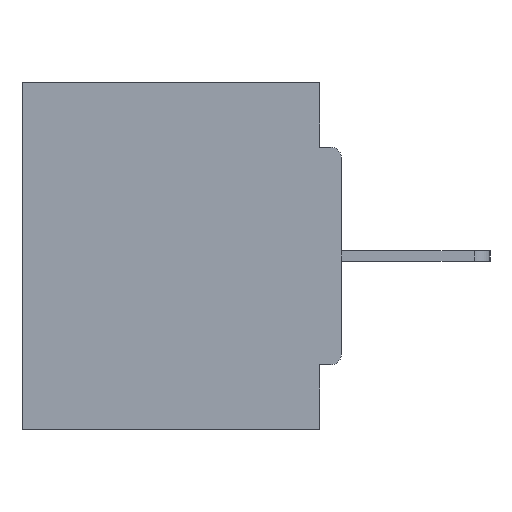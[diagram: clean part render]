
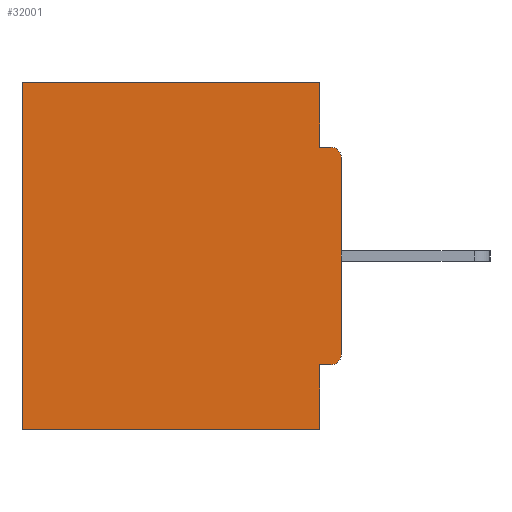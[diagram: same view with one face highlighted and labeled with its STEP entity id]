
A CAD part, left-side view. The second image highlights one B-rep face of the part: STEP entity #32001.
In plain terms, the highlighted planar face has unit normal (-1, 0, 0).
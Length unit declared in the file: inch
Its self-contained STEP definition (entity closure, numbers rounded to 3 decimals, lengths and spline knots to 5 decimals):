
#364 = DIRECTION ( 'NONE',  ( -1., 0., 0. ) ) ;
#591 = ORIENTED_EDGE ( 'NONE', *, *, #34747, .F. ) ;
#621 = ORIENTED_EDGE ( 'NONE', *, *, #23755, .F. ) ;
#860 = VERTEX_POINT ( 'NONE', #31002 ) ;
#2005 = VERTEX_POINT ( 'NONE', #24879 ) ;
#2079 = VERTEX_POINT ( 'NONE', #33691 ) ;
#2296 = VERTEX_POINT ( 'NONE', #29542 ) ;
#2443 = VECTOR ( 'NONE', #19732, 39.37008 ) ;
#3284 = ORIENTED_EDGE ( 'NONE', *, *, #6980, .F. ) ;
#3591 = CARTESIAN_POINT ( 'NONE',  ( 0.298, 0.015, -0.1085 ) ) ;
#4628 = CARTESIAN_POINT ( 'NONE',  ( 0.298, 0., -0.4065 ) ) ;
#4736 = CARTESIAN_POINT ( 'NONE',  ( 0.298, 0.015, -0.4065 ) ) ;
#5088 = EDGE_CURVE ( 'NONE', #2296, #21589, #22859, .T. ) ;
#5742 = DIRECTION ( 'NONE',  ( 0., 0., -1. ) ) ;
#5996 = CARTESIAN_POINT ( 'NONE',  ( 0.298, 0.015, -0.3915 ) ) ;
#6000 = DIRECTION ( 'NONE',  ( 1., 0., 0. ) ) ;
#6258 = EDGE_CURVE ( 'NONE', #8604, #18274, #10541, .T. ) ;
#6264 = DIRECTION ( 'NONE',  ( 0., 0., -1. ) ) ;
#6980 = EDGE_CURVE ( 'NONE', #11764, #2005, #26445, .T. ) ;
#7114 = AXIS2_PLACEMENT_3D ( 'NONE', #3591, #364, #24873 ) ;
#7462 = ORIENTED_EDGE ( 'NONE', *, *, #21615, .T. ) ;
#7548 = ORIENTED_EDGE ( 'NONE', *, *, #29769, .F. ) ;
#7739 = DIRECTION ( 'NONE',  ( 0., 1., 0. ) ) ;
#8064 = VECTOR ( 'NONE', #6264, 39.37008 ) ;
#8521 = VERTEX_POINT ( 'NONE', #31643 ) ;
#8586 = CARTESIAN_POINT ( 'NONE',  ( 0.298, 0., -0.0935 ) ) ;
#8604 = VERTEX_POINT ( 'NONE', #27797 ) ;
#8620 = VECTOR ( 'NONE', #13738, 39.37008 ) ;
#8694 = CARTESIAN_POINT ( 'NONE',  ( 0.298, 0., 0. ) ) ;
#9532 = CARTESIAN_POINT ( 'NONE',  ( 0.298, 0.46, 0. ) ) ;
#10541 = CIRCLE ( 'NONE', #7114, 0.015 ) ;
#11254 = ORIENTED_EDGE ( 'NONE', *, *, #6258, .T. ) ;
#11764 = VERTEX_POINT ( 'NONE', #4736 ) ;
#11808 = VECTOR ( 'NONE', #5742, 39.37008 ) ;
#12014 = CARTESIAN_POINT ( 'NONE',  ( 0.298, 0.031, -0.5 ) ) ;
#12290 = VECTOR ( 'NONE', #31853, 39.37008 ) ;
#13162 = ORIENTED_EDGE ( 'NONE', *, *, #5088, .T. ) ;
#13738 = DIRECTION ( 'NONE',  ( 0., 1., 0. ) ) ;
#14114 = FACE_OUTER_BOUND ( 'NONE', #22584, .T. ) ;
#15560 = EDGE_CURVE ( 'NONE', #8604, #33678, #20438, .T. ) ;
#16738 = CARTESIAN_POINT ( 'NONE',  ( 0.298, 0.031, -0.5 ) ) ;
#17001 = DIRECTION ( 'NONE',  ( -1., 0., 0. ) ) ;
#17617 = ORIENTED_EDGE ( 'NONE', *, *, #30926, .F. ) ;
#17828 = DIRECTION ( 'NONE',  ( 0., 0., -1. ) ) ;
#17941 = DIRECTION ( 'NONE',  ( 0., 0., -1. ) ) ;
#17947 = CARTESIAN_POINT ( 'NONE',  ( 0.298, 0., -0.3915 ) ) ;
#18274 = VERTEX_POINT ( 'NONE', #24307 ) ;
#18898 = LINE ( 'NONE', #16738, #11808 ) ;
#19152 = DIRECTION ( 'NONE',  ( 0., 0., -1. ) ) ;
#19646 = AXIS2_PLACEMENT_3D ( 'NONE', #5996, #17001, #19152 ) ;
#19732 = DIRECTION ( 'NONE',  ( 0., -1., 0. ) ) ;
#19863 = CARTESIAN_POINT ( 'NONE',  ( 0.298, 0., 0. ) ) ;
#20216 = AXIS2_PLACEMENT_3D ( 'NONE', #19863, #6000, #25125 ) ;
#20438 = LINE ( 'NONE', #34148, #29226 ) ;
#21589 = VERTEX_POINT ( 'NONE', #24380 ) ;
#21615 = EDGE_CURVE ( 'NONE', #2079, #2296, #33394, .T. ) ;
#22476 = LINE ( 'NONE', #12014, #8064 ) ;
#22584 = EDGE_LOOP ( 'NONE', ( #11254, #591, #7548, #7462, #13162, #17617, #621, #3284, #33680, #22994 ) ) ;
#22859 = LINE ( 'NONE', #9532, #28917 ) ;
#22994 = ORIENTED_EDGE ( 'NONE', *, *, #15560, .F. ) ;
#23626 = LINE ( 'NONE', #26330, #26528 ) ;
#23755 = EDGE_CURVE ( 'NONE', #2005, #8521, #22476, .T. ) ;
#24307 = CARTESIAN_POINT ( 'NONE',  ( 0.298, 0.015, -0.0935 ) ) ;
#24380 = CARTESIAN_POINT ( 'NONE',  ( 0.298, 0.46, -0.5 ) ) ;
#24873 = DIRECTION ( 'NONE',  ( 0., 0., -1. ) ) ;
#24879 = CARTESIAN_POINT ( 'NONE',  ( 0.298, 0.031, -0.4065 ) ) ;
#25125 = DIRECTION ( 'NONE',  ( 0., 0., -1. ) ) ;
#25298 = PLANE ( 'NONE',  #20216 ) ;
#26330 = CARTESIAN_POINT ( 'NONE',  ( 0.298, 0., -0.5 ) ) ;
#26445 = LINE ( 'NONE', #4628, #12290 ) ;
#26528 = VECTOR ( 'NONE', #7739, 39.37008 ) ;
#27797 = CARTESIAN_POINT ( 'NONE',  ( 0.298, 0., -0.1085 ) ) ;
#28059 = LINE ( 'NONE', #8586, #2443 ) ;
#28917 = VECTOR ( 'NONE', #17828, 39.37008 ) ;
#29226 = VECTOR ( 'NONE', #17941, 39.37008 ) ;
#29542 = CARTESIAN_POINT ( 'NONE',  ( 0.298, 0.46, 0. ) ) ;
#29769 = EDGE_CURVE ( 'NONE', #2079, #860, #18898, .T. ) ;
#30926 = EDGE_CURVE ( 'NONE', #8521, #21589, #23626, .T. ) ;
#31002 = CARTESIAN_POINT ( 'NONE',  ( 0.298, 0.031, -0.0935 ) ) ;
#31643 = CARTESIAN_POINT ( 'NONE',  ( 0.298, 0.031, -0.5 ) ) ;
#31853 = DIRECTION ( 'NONE',  ( 0., 1., 0. ) ) ;
#32001 = ADVANCED_FACE ( 'NONE', ( #14114 ), #25298, .F. ) ;
#32322 = CIRCLE ( 'NONE', #19646, 0.015 ) ;
#33394 = LINE ( 'NONE', #8694, #8620 ) ;
#33678 = VERTEX_POINT ( 'NONE', #17947 ) ;
#33680 = ORIENTED_EDGE ( 'NONE', *, *, #34052, .T. ) ;
#33691 = CARTESIAN_POINT ( 'NONE',  ( 0.298, 0.031, 0. ) ) ;
#34052 = EDGE_CURVE ( 'NONE', #11764, #33678, #32322, .T. ) ;
#34148 = CARTESIAN_POINT ( 'NONE',  ( 0.298, 0., 0. ) ) ;
#34747 = EDGE_CURVE ( 'NONE', #860, #18274, #28059, .T. ) ;
